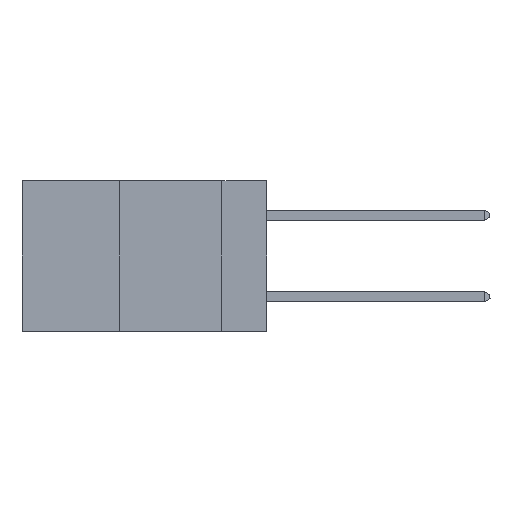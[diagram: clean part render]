
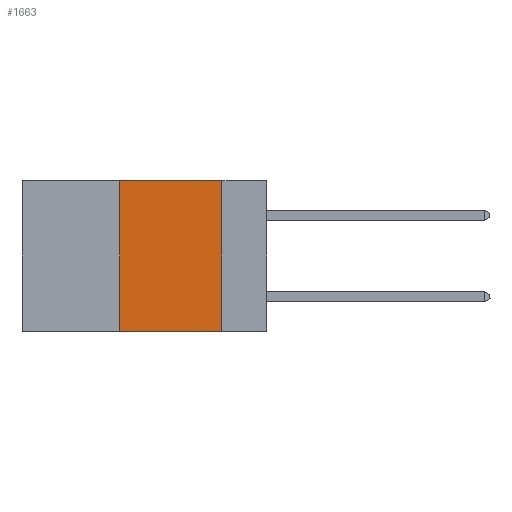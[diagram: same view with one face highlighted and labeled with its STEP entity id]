
A CAD part, left-side view. The second image highlights one B-rep face of the part: STEP entity #1663.
In plain terms, the highlighted planar face has unit normal (-1, 0, 0).
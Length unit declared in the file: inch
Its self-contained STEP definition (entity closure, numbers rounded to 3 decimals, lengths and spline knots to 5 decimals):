
#19 = EDGE_CURVE ( 'NONE', #12209, #9573, #13707, .T. ) ;
#256 = DIRECTION ( 'NONE',  ( 0., 0., -1. ) ) ;
#700 = DIRECTION ( 'NONE',  ( 0., 0., -1. ) ) ;
#893 = EDGE_LOOP ( 'NONE', ( #14563, #13815, #7693, #6520 ) ) ;
#962 = FACE_OUTER_BOUND ( 'NONE', #893, .T. ) ;
#1560 = DIRECTION ( 'NONE',  ( 0., 0., 1. ) ) ;
#1663 = ADVANCED_FACE ( 'NONE', ( #962 ), #5408, .F. ) ;
#1728 = VERTEX_POINT ( 'NONE', #22110 ) ;
#1740 = VECTOR ( 'NONE', #19345, 39.37008 ) ;
#3146 = CARTESIAN_POINT ( 'NONE',  ( 0., 0.6, 0. ) ) ;
#3262 = EDGE_CURVE ( 'NONE', #19747, #12209, #14706, .T. ) ;
#4166 = CARTESIAN_POINT ( 'NONE',  ( 0., 0.11, 0. ) ) ;
#5408 = PLANE ( 'NONE',  #8552 ) ;
#5421 = CARTESIAN_POINT ( 'NONE',  ( 0., 0.36, 0. ) ) ;
#6016 = CARTESIAN_POINT ( 'NONE',  ( 0., 0.11, -0.37 ) ) ;
#6520 = ORIENTED_EDGE ( 'NONE', *, *, #22048, .T. ) ;
#6718 = LINE ( 'NONE', #5421, #19097 ) ;
#7686 = VECTOR ( 'NONE', #21512, 39.37008 ) ;
#7693 = ORIENTED_EDGE ( 'NONE', *, *, #17825, .F. ) ;
#8552 = AXIS2_PLACEMENT_3D ( 'NONE', #9302, #14528, #256 ) ;
#9302 = CARTESIAN_POINT ( 'NONE',  ( 0., 0.6, 0. ) ) ;
#9573 = VERTEX_POINT ( 'NONE', #6016 ) ;
#10723 = CARTESIAN_POINT ( 'NONE',  ( 0., 0.36, 0. ) ) ;
#10745 = CARTESIAN_POINT ( 'NONE',  ( 0., 0.6, -0.37 ) ) ;
#11869 = LINE ( 'NONE', #10745, #7686 ) ;
#12209 = VERTEX_POINT ( 'NONE', #4166 ) ;
#13707 = LINE ( 'NONE', #19867, #15419 ) ;
#13815 = ORIENTED_EDGE ( 'NONE', *, *, #3262, .F. ) ;
#14528 = DIRECTION ( 'NONE',  ( 1., 0., 0. ) ) ;
#14563 = ORIENTED_EDGE ( 'NONE', *, *, #19, .F. ) ;
#14706 = LINE ( 'NONE', #3146, #1740 ) ;
#15419 = VECTOR ( 'NONE', #700, 39.37008 ) ;
#17825 = EDGE_CURVE ( 'NONE', #1728, #19747, #6718, .T. ) ;
#19097 = VECTOR ( 'NONE', #1560, 39.37008 ) ;
#19345 = DIRECTION ( 'NONE',  ( 0., -1., 0. ) ) ;
#19747 = VERTEX_POINT ( 'NONE', #10723 ) ;
#19867 = CARTESIAN_POINT ( 'NONE',  ( 0., 0.11, 0. ) ) ;
#21512 = DIRECTION ( 'NONE',  ( 0., -1., 0. ) ) ;
#22048 = EDGE_CURVE ( 'NONE', #1728, #9573, #11869, .T. ) ;
#22110 = CARTESIAN_POINT ( 'NONE',  ( 0., 0.36, -0.37 ) ) ;
